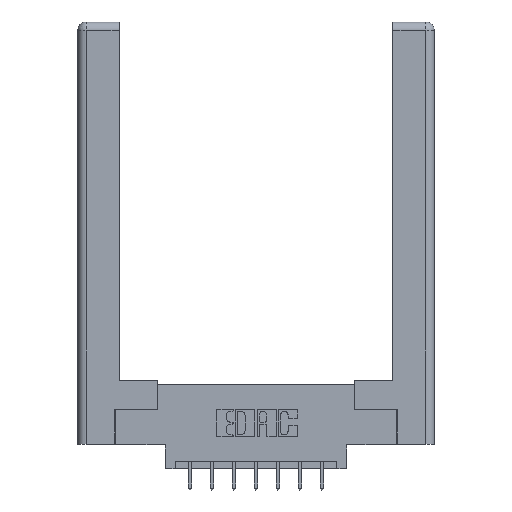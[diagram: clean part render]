
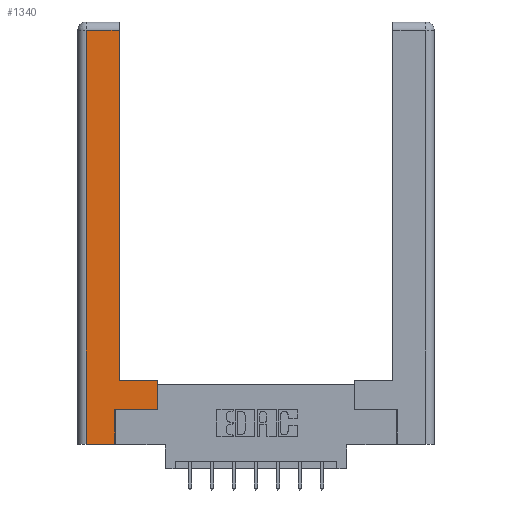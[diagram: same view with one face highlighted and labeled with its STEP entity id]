
A CAD part, top view. The second image highlights one B-rep face of the part: STEP entity #1340.
In plain terms, the highlighted planar face has unit normal (0, 0, 1).
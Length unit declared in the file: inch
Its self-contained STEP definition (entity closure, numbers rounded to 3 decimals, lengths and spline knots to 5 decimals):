
#59 = ORIENTED_EDGE ( 'NONE', *, *, #4793, .T. ) ;
#122 = LINE ( 'NONE', #10015, #2441 ) ;
#148 = CARTESIAN_POINT ( 'NONE',  ( 0.265, 0.245, 0. ) ) ;
#302 = LINE ( 'NONE', #9104, #467 ) ;
#412 = VERTEX_POINT ( 'NONE', #6093 ) ;
#467 = VECTOR ( 'NONE', #4197, 39.37008 ) ;
#633 = VECTOR ( 'NONE', #5519, 39.37008 ) ;
#747 = CARTESIAN_POINT ( 'NONE',  ( 0.265, 0., 0. ) ) ;
#1107 = DIRECTION ( 'NONE',  ( 0., 1., 0. ) ) ;
#1178 = VERTEX_POINT ( 'NONE', #148 ) ;
#1340 = ADVANCED_FACE ( 'NONE', ( #1429 ), #2271, .F. ) ;
#1429 = FACE_OUTER_BOUND ( 'NONE', #2473, .T. ) ;
#1510 = ORIENTED_EDGE ( 'NONE', *, *, #2902, .T. ) ;
#1683 = ORIENTED_EDGE ( 'NONE', *, *, #3421, .T. ) ;
#2104 = DIRECTION ( 'NONE',  ( 0., 0., -1. ) ) ;
#2271 = PLANE ( 'NONE',  #8728 ) ;
#2317 = CARTESIAN_POINT ( 'NONE',  ( 0.565, 0.245, 0. ) ) ;
#2441 = VECTOR ( 'NONE', #10964, 39.37008 ) ;
#2473 = EDGE_LOOP ( 'NONE', ( #6475, #59, #1510, #11935, #2942, #2571, #1683, #7530 ) ) ;
#2533 = LINE ( 'NONE', #2317, #4073 ) ;
#2571 = ORIENTED_EDGE ( 'NONE', *, *, #6177, .T. ) ;
#2646 = EDGE_CURVE ( 'NONE', #11303, #6977, #9566, .T. ) ;
#2898 = VERTEX_POINT ( 'NONE', #747 ) ;
#2902 = EDGE_CURVE ( 'NONE', #4583, #412, #6313, .T. ) ;
#2942 = ORIENTED_EDGE ( 'NONE', *, *, #9441, .T. ) ;
#3421 = EDGE_CURVE ( 'NONE', #6160, #11303, #302, .T. ) ;
#3479 = DIRECTION ( 'NONE',  ( 1., 0., 0. ) ) ;
#4073 = VECTOR ( 'NONE', #3479, 39.37008 ) ;
#4197 = DIRECTION ( 'NONE',  ( 0., 1., 0. ) ) ;
#4252 = EDGE_CURVE ( 'NONE', #412, #2898, #122, .T. ) ;
#4583 = VERTEX_POINT ( 'NONE', #6046 ) ;
#4738 = CARTESIAN_POINT ( 'NONE',  ( 0.295, 0.45, 0. ) ) ;
#4793 = EDGE_CURVE ( 'NONE', #10294, #4583, #7351, .T. ) ;
#4835 = DIRECTION ( 'NONE',  ( 0., 1., 0. ) ) ;
#5132 = CARTESIAN_POINT ( 'NONE',  ( 0.565, 0.45, 0. ) ) ;
#5168 = CARTESIAN_POINT ( 'NONE',  ( 0.265, 0.245, 0. ) ) ;
#5519 = DIRECTION ( 'NONE',  ( -1., 0., 0. ) ) ;
#5984 = VECTOR ( 'NONE', #11291, 39.37008 ) ;
#5986 = DIRECTION ( 'NONE',  ( -1., 0., 0. ) ) ;
#6046 = CARTESIAN_POINT ( 'NONE',  ( 0.0615, 2.94, 0. ) ) ;
#6093 = CARTESIAN_POINT ( 'NONE',  ( 0.0615, 0., 0. ) ) ;
#6160 = VERTEX_POINT ( 'NONE', #7161 ) ;
#6177 = EDGE_CURVE ( 'NONE', #1178, #6160, #2533, .T. ) ;
#6313 = LINE ( 'NONE', #9330, #5984 ) ;
#6475 = ORIENTED_EDGE ( 'NONE', *, *, #8392, .T. ) ;
#6676 = LINE ( 'NONE', #5168, #10538 ) ;
#6977 = VERTEX_POINT ( 'NONE', #4738 ) ;
#7161 = CARTESIAN_POINT ( 'NONE',  ( 0.565, 0.245, 0. ) ) ;
#7351 = LINE ( 'NONE', #12617, #10117 ) ;
#7439 = CARTESIAN_POINT ( 'NONE',  ( 0.295, 2.94, 0. ) ) ;
#7530 = ORIENTED_EDGE ( 'NONE', *, *, #2646, .T. ) ;
#8108 = CARTESIAN_POINT ( 'NONE',  ( 0., 0., 0. ) ) ;
#8392 = EDGE_CURVE ( 'NONE', #6977, #10294, #8716, .T. ) ;
#8716 = LINE ( 'NONE', #10754, #11474 ) ;
#8728 = AXIS2_PLACEMENT_3D ( 'NONE', #8108, #2104, #5986 ) ;
#9104 = CARTESIAN_POINT ( 'NONE',  ( 0.565, 0.45, 0. ) ) ;
#9330 = CARTESIAN_POINT ( 'NONE',  ( 0.0615, 0., 0. ) ) ;
#9441 = EDGE_CURVE ( 'NONE', #2898, #1178, #6676, .T. ) ;
#9561 = DIRECTION ( 'NONE',  ( -1., 0., 0. ) ) ;
#9566 = LINE ( 'NONE', #11286, #633 ) ;
#10015 = CARTESIAN_POINT ( 'NONE',  ( 0.265, 0., 0. ) ) ;
#10117 = VECTOR ( 'NONE', #9561, 39.37008 ) ;
#10294 = VERTEX_POINT ( 'NONE', #7439 ) ;
#10538 = VECTOR ( 'NONE', #1107, 39.37008 ) ;
#10754 = CARTESIAN_POINT ( 'NONE',  ( 0.295, 3., 0. ) ) ;
#10964 = DIRECTION ( 'NONE',  ( 1., 0., 0. ) ) ;
#11286 = CARTESIAN_POINT ( 'NONE',  ( 0.295, 0.45, 0. ) ) ;
#11291 = DIRECTION ( 'NONE',  ( 0., -1., 0. ) ) ;
#11303 = VERTEX_POINT ( 'NONE', #5132 ) ;
#11474 = VECTOR ( 'NONE', #4835, 39.37008 ) ;
#11935 = ORIENTED_EDGE ( 'NONE', *, *, #4252, .T. ) ;
#12617 = CARTESIAN_POINT ( 'NONE',  ( 0.0615, 2.94, 0. ) ) ;
